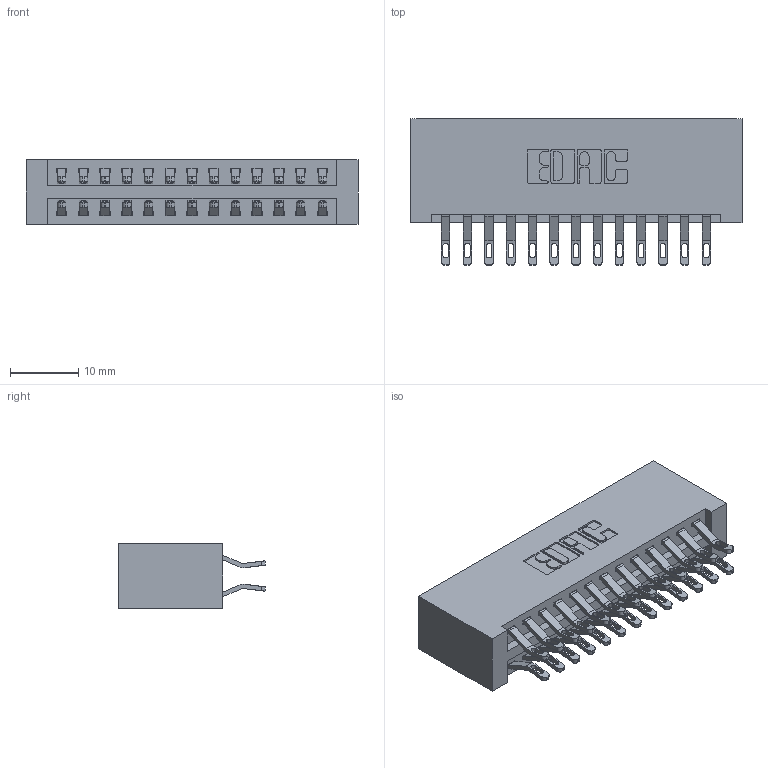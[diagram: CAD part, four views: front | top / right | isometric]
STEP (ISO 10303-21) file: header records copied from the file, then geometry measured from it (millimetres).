
FILE_DESCRIPTION (( 'STEP AP203' ), '1' );
FILE_NAME ('346-026-555-201.STEP', '2018-08-21T22:57:34', ( '' ), ( '' ), 'SwSTEP 2.0', 'SolidWorks 2016', '' );
FILE_SCHEMA (( 'CONFIG_CONTROL_DESIGN' ));
Length unit declared in the file: inch
Products named in the file (3): 346 Part_No Mounting Lugs; 345-292-001_555 Tail; 346-026-555-201
Assembly tree (27 placements, depth 2):
  346-026-555-201
    346 Part_No Mounting Lugs
    345-292-001_555 Tail  x26
Bounding box: 48.51 x 21.46 x 9.4 mm (x, y, z)
Volume: 5154.2 mm3; surface area: 7061 mm2
Topology: 27 solids, 27 shells, 1622 faces, 5063 edges, 3374 vertices
Faces by surface type: plane 930, cylinder 692
Entity records: 12437 total; most frequent: CARTESIAN_POINT 2122, ORIENTED_EDGE 2026, DIRECTION 1885, EDGE_CURVE 1013, LINE 817, VECTOR 817, VERTEX_POINT 674, AXIS2_PLACEMENT_3D 534
